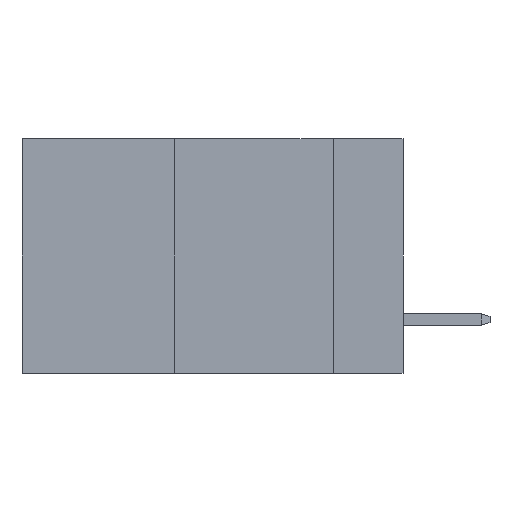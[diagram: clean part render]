
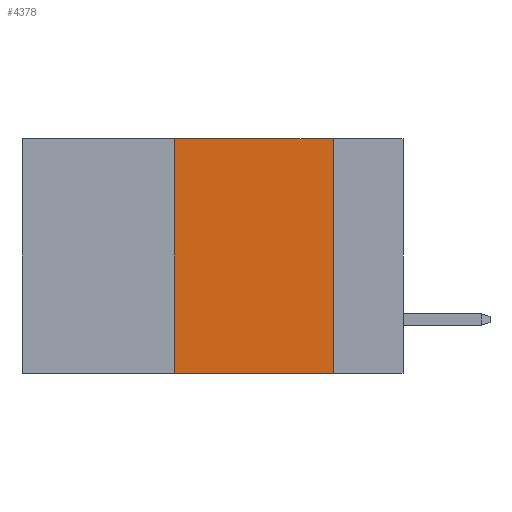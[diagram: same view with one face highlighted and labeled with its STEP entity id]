
A CAD part, left-side view. The second image highlights one B-rep face of the part: STEP entity #4378.
In plain terms, the highlighted planar face has unit normal (-1, 0, 0).
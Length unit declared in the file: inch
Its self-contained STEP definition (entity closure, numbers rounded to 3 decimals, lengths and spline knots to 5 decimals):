
#959 = ORIENTED_EDGE ( 'NONE', *, *, #14229, .F. ) ;
#1399 = CARTESIAN_POINT ( 'NONE',  ( 0., 0.11, 0. ) ) ;
#1696 = DIRECTION ( 'NONE',  ( 0., 0., -1. ) ) ;
#2083 = VERTEX_POINT ( 'NONE', #8724 ) ;
#3543 = LINE ( 'NONE', #11438, #14629 ) ;
#3642 = DIRECTION ( 'NONE',  ( 0., -1., 0. ) ) ;
#4282 = ORIENTED_EDGE ( 'NONE', *, *, #7992, .F. ) ;
#4378 = ADVANCED_FACE ( 'NONE', ( #7828 ), #9107, .F. ) ;
#4923 = CARTESIAN_POINT ( 'NONE',  ( 0., 0.36, 0. ) ) ;
#5022 = CARTESIAN_POINT ( 'NONE',  ( 0., 0.6, -0.37 ) ) ;
#5167 = LINE ( 'NONE', #10476, #9185 ) ;
#5490 = VECTOR ( 'NONE', #10487, 39.37008 ) ;
#6545 = LINE ( 'NONE', #11689, #5490 ) ;
#7406 = DIRECTION ( 'NONE',  ( 0., -1., 0. ) ) ;
#7506 = LINE ( 'NONE', #5022, #8798 ) ;
#7607 = ORIENTED_EDGE ( 'NONE', *, *, #9202, .T. ) ;
#7828 = FACE_OUTER_BOUND ( 'NONE', #14545, .T. ) ;
#7992 = EDGE_CURVE ( 'NONE', #9288, #8061, #3543, .T. ) ;
#8061 = VERTEX_POINT ( 'NONE', #1399 ) ;
#8206 = DIRECTION ( 'NONE',  ( 1., 0., 0. ) ) ;
#8724 = CARTESIAN_POINT ( 'NONE',  ( 0., 0.36, -0.37 ) ) ;
#8798 = VECTOR ( 'NONE', #3642, 39.37008 ) ;
#8900 = CARTESIAN_POINT ( 'NONE',  ( 0., 0.11, -0.37 ) ) ;
#9107 = PLANE ( 'NONE',  #11262 ) ;
#9185 = VECTOR ( 'NONE', #12788, 39.37008 ) ;
#9202 = EDGE_CURVE ( 'NONE', #2083, #13762, #7506, .T. ) ;
#9288 = VERTEX_POINT ( 'NONE', #4923 ) ;
#10476 = CARTESIAN_POINT ( 'NONE',  ( 0., 0.36, 0. ) ) ;
#10487 = DIRECTION ( 'NONE',  ( 0., 0., -1. ) ) ;
#11262 = AXIS2_PLACEMENT_3D ( 'NONE', #11688, #8206, #1696 ) ;
#11438 = CARTESIAN_POINT ( 'NONE',  ( 0., 0.6, 0. ) ) ;
#11688 = CARTESIAN_POINT ( 'NONE',  ( 0., 0.6, 0. ) ) ;
#11689 = CARTESIAN_POINT ( 'NONE',  ( 0., 0.11, 0. ) ) ;
#12432 = EDGE_CURVE ( 'NONE', #2083, #9288, #5167, .T. ) ;
#12788 = DIRECTION ( 'NONE',  ( 0., 0., 1. ) ) ;
#13762 = VERTEX_POINT ( 'NONE', #8900 ) ;
#14229 = EDGE_CURVE ( 'NONE', #8061, #13762, #6545, .T. ) ;
#14545 = EDGE_LOOP ( 'NONE', ( #959, #4282, #15976, #7607 ) ) ;
#14629 = VECTOR ( 'NONE', #7406, 39.37008 ) ;
#15976 = ORIENTED_EDGE ( 'NONE', *, *, #12432, .F. ) ;
